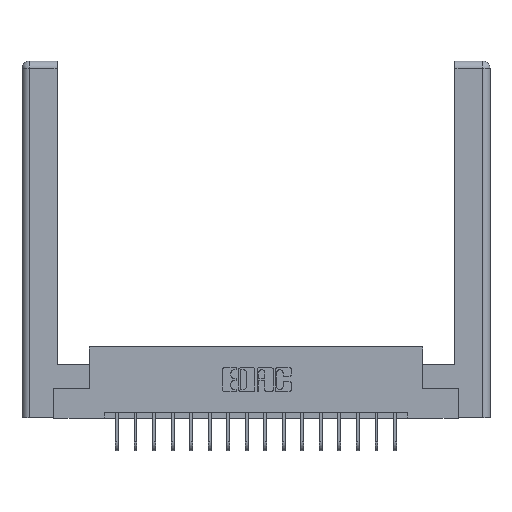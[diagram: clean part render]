
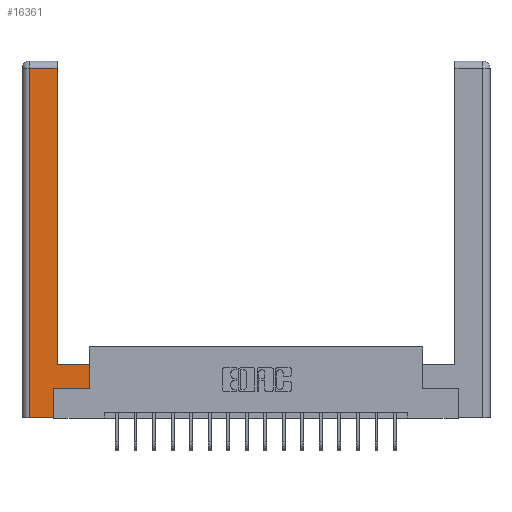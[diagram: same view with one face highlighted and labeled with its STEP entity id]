
A CAD part, top view. The second image highlights one B-rep face of the part: STEP entity #16361.
In plain terms, the highlighted planar face has unit normal (0, 0, 1).
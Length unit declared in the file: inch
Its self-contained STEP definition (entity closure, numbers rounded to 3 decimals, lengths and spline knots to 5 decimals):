
#298 = LINE ( 'NONE', #17934, #10955 ) ;
#536 = CARTESIAN_POINT ( 'NONE',  ( 0.565, 0.45, 0. ) ) ;
#728 = ORIENTED_EDGE ( 'NONE', *, *, #13068, .T. ) ;
#927 = LINE ( 'NONE', #12086, #5241 ) ;
#1299 = VERTEX_POINT ( 'NONE', #14919 ) ;
#1310 = DIRECTION ( 'NONE',  ( -1., 0., 0. ) ) ;
#2598 = VERTEX_POINT ( 'NONE', #16339 ) ;
#2606 = ORIENTED_EDGE ( 'NONE', *, *, #3558, .T. ) ;
#2811 = VECTOR ( 'NONE', #15555, 39.37008 ) ;
#3062 = DIRECTION ( 'NONE',  ( 0., 1., 0. ) ) ;
#3321 = DIRECTION ( 'NONE',  ( 1., 0., 0. ) ) ;
#3454 = DIRECTION ( 'NONE',  ( 0., 1., 0. ) ) ;
#3558 = EDGE_CURVE ( 'NONE', #16004, #13214, #15937, .T. ) ;
#3616 = DIRECTION ( 'NONE',  ( 0., 1., 0. ) ) ;
#3625 = CARTESIAN_POINT ( 'NONE',  ( 0.265, 0.245, 0. ) ) ;
#4685 = VERTEX_POINT ( 'NONE', #6076 ) ;
#5114 = CARTESIAN_POINT ( 'NONE',  ( 0.565, 0.245, 0. ) ) ;
#5163 = ORIENTED_EDGE ( 'NONE', *, *, #5409, .T. ) ;
#5241 = VECTOR ( 'NONE', #3616, 39.37008 ) ;
#5409 = EDGE_CURVE ( 'NONE', #1299, #4685, #13648, .T. ) ;
#6076 = CARTESIAN_POINT ( 'NONE',  ( 0.565, 0.45, 0. ) ) ;
#6339 = VECTOR ( 'NONE', #12011, 39.37008 ) ;
#6659 = LINE ( 'NONE', #3625, #16207 ) ;
#6888 = PLANE ( 'NONE',  #14649 ) ;
#7041 = ORIENTED_EDGE ( 'NONE', *, *, #12435, .T. ) ;
#7154 = LINE ( 'NONE', #8363, #2811 ) ;
#8165 = CARTESIAN_POINT ( 'NONE',  ( 0.265, 0., 0. ) ) ;
#8363 = CARTESIAN_POINT ( 'NONE',  ( 0.0615, 0., 0. ) ) ;
#9300 = VECTOR ( 'NONE', #3062, 39.37008 ) ;
#9448 = CARTESIAN_POINT ( 'NONE',  ( 0.295, 0.45, 0. ) ) ;
#9513 = VECTOR ( 'NONE', #16353, 39.37008 ) ;
#9792 = CARTESIAN_POINT ( 'NONE',  ( 0.0615, 0., 0. ) ) ;
#10955 = VECTOR ( 'NONE', #11155, 39.37008 ) ;
#11116 = VERTEX_POINT ( 'NONE', #14269 ) ;
#11155 = DIRECTION ( 'NONE',  ( -1., 0., 0. ) ) ;
#12011 = DIRECTION ( 'NONE',  ( 1., 0., 0. ) ) ;
#12086 = CARTESIAN_POINT ( 'NONE',  ( 0.295, 3., 0. ) ) ;
#12103 = EDGE_CURVE ( 'NONE', #11116, #2598, #298, .T. ) ;
#12435 = EDGE_CURVE ( 'NONE', #17199, #11116, #927, .T. ) ;
#12498 = DIRECTION ( 'NONE',  ( 0., 0., -1. ) ) ;
#12695 = ORIENTED_EDGE ( 'NONE', *, *, #13606, .T. ) ;
#13067 = CARTESIAN_POINT ( 'NONE',  ( 0.265, 0., 0. ) ) ;
#13068 = EDGE_CURVE ( 'NONE', #14118, #1299, #13721, .T. ) ;
#13160 = VECTOR ( 'NONE', #3321, 39.37008 ) ;
#13214 = VERTEX_POINT ( 'NONE', #8165 ) ;
#13606 = EDGE_CURVE ( 'NONE', #2598, #16004, #7154, .T. ) ;
#13648 = LINE ( 'NONE', #536, #9300 ) ;
#13721 = LINE ( 'NONE', #5114, #6339 ) ;
#14118 = VERTEX_POINT ( 'NONE', #17921 ) ;
#14269 = CARTESIAN_POINT ( 'NONE',  ( 0.295, 2.94, 0. ) ) ;
#14425 = EDGE_LOOP ( 'NONE', ( #7041, #15576, #12695, #2606, #17518, #728, #5163, #15409 ) ) ;
#14526 = LINE ( 'NONE', #9448, #9513 ) ;
#14649 = AXIS2_PLACEMENT_3D ( 'NONE', #15020, #12498, #1310 ) ;
#14919 = CARTESIAN_POINT ( 'NONE',  ( 0.565, 0.245, 0. ) ) ;
#15020 = CARTESIAN_POINT ( 'NONE',  ( 0., 0., 0. ) ) ;
#15180 = EDGE_CURVE ( 'NONE', #4685, #17199, #14526, .T. ) ;
#15409 = ORIENTED_EDGE ( 'NONE', *, *, #15180, .T. ) ;
#15555 = DIRECTION ( 'NONE',  ( 0., -1., 0. ) ) ;
#15576 = ORIENTED_EDGE ( 'NONE', *, *, #12103, .T. ) ;
#15937 = LINE ( 'NONE', #13067, #13160 ) ;
#16004 = VERTEX_POINT ( 'NONE', #9792 ) ;
#16040 = CARTESIAN_POINT ( 'NONE',  ( 0.295, 0.45, 0. ) ) ;
#16207 = VECTOR ( 'NONE', #3454, 39.37008 ) ;
#16238 = EDGE_CURVE ( 'NONE', #13214, #14118, #6659, .T. ) ;
#16339 = CARTESIAN_POINT ( 'NONE',  ( 0.0615, 2.94, 0. ) ) ;
#16353 = DIRECTION ( 'NONE',  ( -1., 0., 0. ) ) ;
#16361 = ADVANCED_FACE ( 'NONE', ( #16850 ), #6888, .F. ) ;
#16850 = FACE_OUTER_BOUND ( 'NONE', #14425, .T. ) ;
#17199 = VERTEX_POINT ( 'NONE', #16040 ) ;
#17518 = ORIENTED_EDGE ( 'NONE', *, *, #16238, .T. ) ;
#17921 = CARTESIAN_POINT ( 'NONE',  ( 0.265, 0.245, 0. ) ) ;
#17934 = CARTESIAN_POINT ( 'NONE',  ( 0.0615, 2.94, 0. ) ) ;
